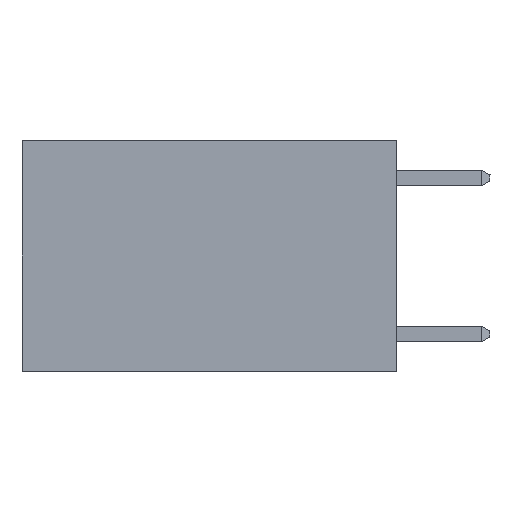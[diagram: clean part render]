
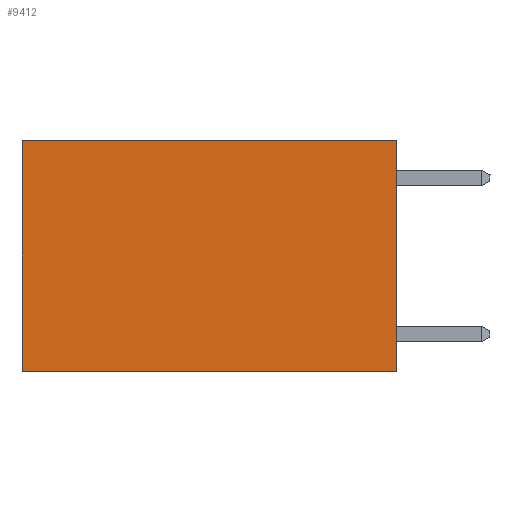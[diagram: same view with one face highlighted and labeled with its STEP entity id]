
A CAD part, left-side view. The second image highlights one B-rep face of the part: STEP entity #9412.
In plain terms, the highlighted planar face has unit normal (-1, 0, 0).
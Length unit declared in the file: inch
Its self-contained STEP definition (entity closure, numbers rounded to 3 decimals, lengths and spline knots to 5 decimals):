
#691 = VECTOR ( 'NONE', #14161, 39.37008 ) ;
#863 = VERTEX_POINT ( 'NONE', #3667 ) ;
#1350 = CARTESIAN_POINT ( 'NONE',  ( 0.2625, 0., 0. ) ) ;
#1549 = CARTESIAN_POINT ( 'NONE',  ( 0.2625, 0., -0.37 ) ) ;
#1575 = LINE ( 'NONE', #10671, #691 ) ;
#1996 = DIRECTION ( 'NONE',  ( 0., 0., -1. ) ) ;
#2072 = EDGE_LOOP ( 'NONE', ( #10386, #2430, #4327, #9908 ) ) ;
#2430 = ORIENTED_EDGE ( 'NONE', *, *, #7651, .F. ) ;
#2707 = EDGE_CURVE ( 'NONE', #7767, #8600, #4730, .T. ) ;
#3133 = CARTESIAN_POINT ( 'NONE',  ( 0.2625, 0., 0. ) ) ;
#3667 = CARTESIAN_POINT ( 'NONE',  ( 0.2625, 0.6, 0. ) ) ;
#4321 = CARTESIAN_POINT ( 'NONE',  ( 0.2625, 0.6, 0. ) ) ;
#4327 = ORIENTED_EDGE ( 'NONE', *, *, #2707, .F. ) ;
#4730 = LINE ( 'NONE', #1350, #9097 ) ;
#4976 = DIRECTION ( 'NONE',  ( 0., 1., 0. ) ) ;
#4977 = VERTEX_POINT ( 'NONE', #7133 ) ;
#5260 = CARTESIAN_POINT ( 'NONE',  ( 0.2625, 0., 0. ) ) ;
#5271 = EDGE_CURVE ( 'NONE', #863, #4977, #12192, .T. ) ;
#5391 = CARTESIAN_POINT ( 'NONE',  ( 0.2625, 0., -0.37 ) ) ;
#5965 = DIRECTION ( 'NONE',  ( 0., 0., -1. ) ) ;
#6592 = DIRECTION ( 'NONE',  ( 1., 0., 0. ) ) ;
#7133 = CARTESIAN_POINT ( 'NONE',  ( 0.2625, 0.6, -0.37 ) ) ;
#7651 = EDGE_CURVE ( 'NONE', #8600, #4977, #11679, .T. ) ;
#7731 = PLANE ( 'NONE',  #13508 ) ;
#7767 = VERTEX_POINT ( 'NONE', #3133 ) ;
#8600 = VERTEX_POINT ( 'NONE', #5391 ) ;
#8950 = DIRECTION ( 'NONE',  ( 0., 0., -1. ) ) ;
#9097 = VECTOR ( 'NONE', #5965, 39.37008 ) ;
#9412 = ADVANCED_FACE ( 'NONE', ( #10043 ), #7731, .F. ) ;
#9908 = ORIENTED_EDGE ( 'NONE', *, *, #11763, .T. ) ;
#10043 = FACE_OUTER_BOUND ( 'NONE', #2072, .T. ) ;
#10193 = VECTOR ( 'NONE', #1996, 39.37008 ) ;
#10386 = ORIENTED_EDGE ( 'NONE', *, *, #5271, .T. ) ;
#10671 = CARTESIAN_POINT ( 'NONE',  ( 0.2625, 0., 0. ) ) ;
#11679 = LINE ( 'NONE', #1549, #13638 ) ;
#11763 = EDGE_CURVE ( 'NONE', #7767, #863, #1575, .T. ) ;
#12192 = LINE ( 'NONE', #4321, #10193 ) ;
#13508 = AXIS2_PLACEMENT_3D ( 'NONE', #5260, #6592, #8950 ) ;
#13638 = VECTOR ( 'NONE', #4976, 39.37008 ) ;
#14161 = DIRECTION ( 'NONE',  ( 0., 1., 0. ) ) ;
